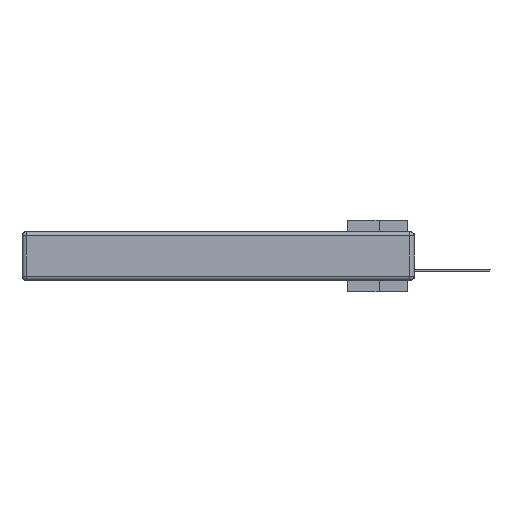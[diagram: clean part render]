
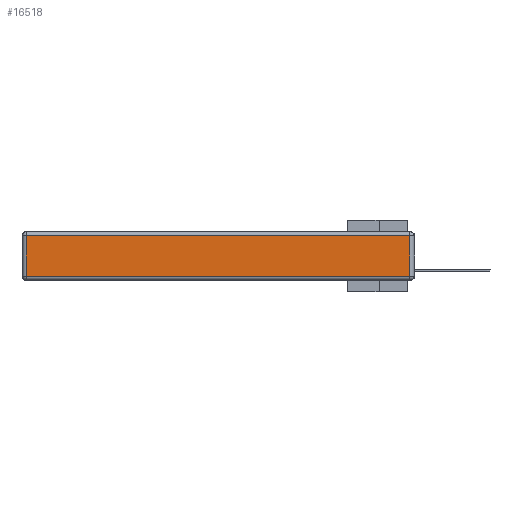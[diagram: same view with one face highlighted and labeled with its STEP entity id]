
A CAD part, left-side view. The second image highlights one B-rep face of the part: STEP entity #16518.
In plain terms, the highlighted planar face has unit normal (-1, 0, 0).
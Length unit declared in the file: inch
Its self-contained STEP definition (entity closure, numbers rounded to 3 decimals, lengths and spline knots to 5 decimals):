
#1031 = DIRECTION ( 'NONE',  ( 0., 0., 1. ) ) ;
#2165 = CARTESIAN_POINT ( 'NONE',  ( 0., 0., -0.343 ) ) ;
#2389 = LINE ( 'NONE', #13426, #28309 ) ;
#3942 = ORIENTED_EDGE ( 'NONE', *, *, #6228, .T. ) ;
#4852 = CARTESIAN_POINT ( 'NONE',  ( 0., 2.72, -0.343 ) ) ;
#4910 = LINE ( 'NONE', #27005, #29627 ) ;
#5396 = DIRECTION ( 'NONE',  ( 0., 0., -1. ) ) ;
#6228 = EDGE_CURVE ( 'NONE', #12412, #30777, #4910, .T. ) ;
#7436 = DIRECTION ( 'NONE',  ( 0., 0., 1. ) ) ;
#8566 = CARTESIAN_POINT ( 'NONE',  ( 0., 0.03, -0.313 ) ) ;
#9327 = DIRECTION ( 'NONE',  ( 0., 1., 0. ) ) ;
#9475 = CARTESIAN_POINT ( 'NONE',  ( 0., 2.72, -0.03 ) ) ;
#9977 = CARTESIAN_POINT ( 'NONE',  ( 0., 2.72, -0.313 ) ) ;
#12302 = VERTEX_POINT ( 'NONE', #9977 ) ;
#12412 = VERTEX_POINT ( 'NONE', #13585 ) ;
#12474 = FACE_OUTER_BOUND ( 'NONE', #24363, .T. ) ;
#12663 = PLANE ( 'NONE',  #14907 ) ;
#13426 = CARTESIAN_POINT ( 'NONE',  ( 0., 0., -0.313 ) ) ;
#13462 = ORIENTED_EDGE ( 'NONE', *, *, #22691, .T. ) ;
#13585 = CARTESIAN_POINT ( 'NONE',  ( 0., 0.03, -0.03 ) ) ;
#14907 = AXIS2_PLACEMENT_3D ( 'NONE', #2165, #31695, #7436 ) ;
#16518 = ADVANCED_FACE ( 'NONE', ( #12474 ), #12663, .T. ) ;
#19140 = LINE ( 'NONE', #4852, #30554 ) ;
#21030 = VERTEX_POINT ( 'NONE', #8566 ) ;
#21757 = DIRECTION ( 'NONE',  ( 0., -1., 0. ) ) ;
#22691 = EDGE_CURVE ( 'NONE', #21030, #12412, #31271, .T. ) ;
#24363 = EDGE_LOOP ( 'NONE', ( #33806, #13462, #3942, #31101 ) ) ;
#27005 = CARTESIAN_POINT ( 'NONE',  ( 0., 2.75, -0.03 ) ) ;
#27834 = EDGE_CURVE ( 'NONE', #12302, #21030, #2389, .T. ) ;
#28309 = VECTOR ( 'NONE', #21757, 39.37008 ) ;
#28559 = CARTESIAN_POINT ( 'NONE',  ( 0., 0.03, -0.343 ) ) ;
#29627 = VECTOR ( 'NONE', #9327, 39.37008 ) ;
#30554 = VECTOR ( 'NONE', #5396, 39.37008 ) ;
#30777 = VERTEX_POINT ( 'NONE', #9475 ) ;
#31101 = ORIENTED_EDGE ( 'NONE', *, *, #31814, .T. ) ;
#31271 = LINE ( 'NONE', #28559, #33833 ) ;
#31695 = DIRECTION ( 'NONE',  ( -1., 0., 0. ) ) ;
#31814 = EDGE_CURVE ( 'NONE', #30777, #12302, #19140, .T. ) ;
#33806 = ORIENTED_EDGE ( 'NONE', *, *, #27834, .T. ) ;
#33833 = VECTOR ( 'NONE', #1031, 39.37008 ) ;
